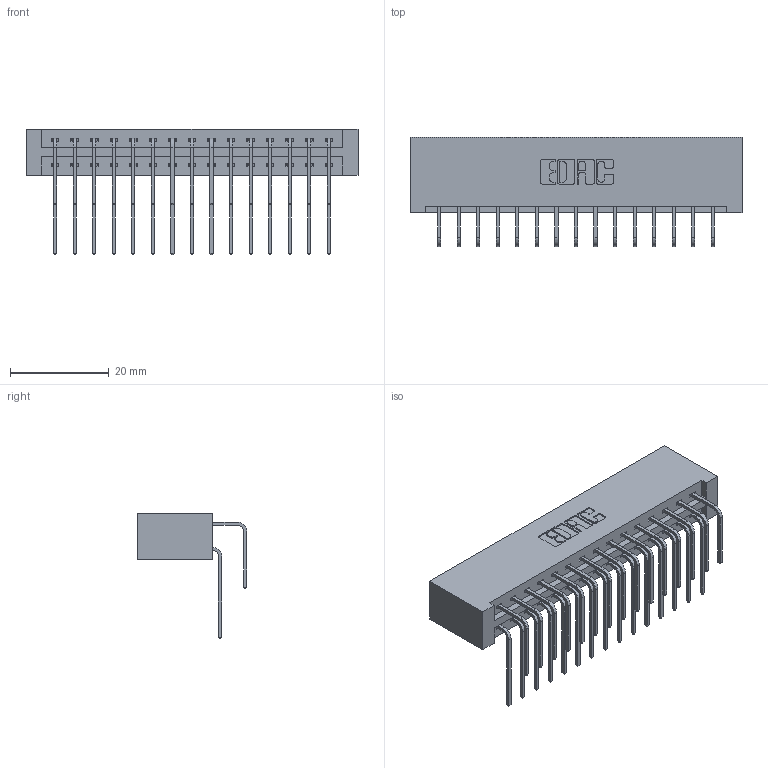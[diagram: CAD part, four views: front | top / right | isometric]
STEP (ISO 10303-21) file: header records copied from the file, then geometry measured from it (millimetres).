
FILE_DESCRIPTION (( 'STEP AP203' ), '1' );
FILE_NAME ('387-030-558-201.STEP', '2019-10-17T15:00:10', ( '' ), ( '' ), 'SwSTEP 2.0', 'SolidWorks 2016', '' );
FILE_SCHEMA (( 'CONFIG_CONTROL_DESIGN' ));
Length unit declared in the file: inch
Products named in the file (4): 337 Part_No Mounting Lugs; 345-292-001_558 559 Tail - 1; 345-292-001_558 Tail - 2; 387-030-558-201
Assembly tree (31 placements, depth 2):
  387-030-558-201
    337 Part_No Mounting Lugs
    345-292-001_558 559 Tail - 1  x15
    345-292-001_558 Tail - 2  x15
Bounding box: 67.31 x 22.17 x 25.53 mm (x, y, z)
Volume: 7668.1 mm3; surface area: 9331.6 mm2
Topology: 31 solids, 31 shells, 1786 faces, 5297 edges, 3490 vertices
Faces by surface type: plane 1266, cylinder 520
Entity records: 16629 total; most frequent: CARTESIAN_POINT 2869, ORIENTED_EDGE 2754, DIRECTION 2465, EDGE_CURVE 1377, LINE 1217, VECTOR 1217, VERTEX_POINT 914, AXIS2_PLACEMENT_3D 624
